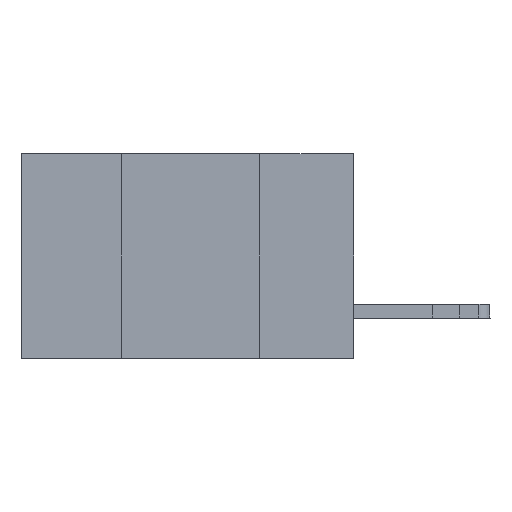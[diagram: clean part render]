
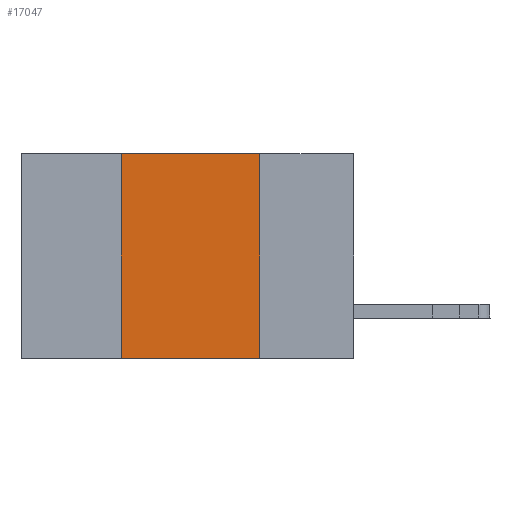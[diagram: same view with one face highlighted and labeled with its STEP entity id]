
A CAD part, left-side view. The second image highlights one B-rep face of the part: STEP entity #17047.
In plain terms, the highlighted planar face has unit normal (-1, 0, 0).
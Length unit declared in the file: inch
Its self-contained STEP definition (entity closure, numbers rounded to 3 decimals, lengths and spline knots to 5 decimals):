
#744 = CARTESIAN_POINT ( 'NONE',  ( 0., 0.42, 0. ) ) ;
#841 = CARTESIAN_POINT ( 'NONE',  ( 0., 0.17, 0. ) ) ;
#2110 = VECTOR ( 'NONE', #11971, 39.37008 ) ;
#2555 = CARTESIAN_POINT ( 'NONE',  ( 0., 0.6, 0. ) ) ;
#3295 = CARTESIAN_POINT ( 'NONE',  ( 0., 0.42, -0.37 ) ) ;
#3347 = FACE_OUTER_BOUND ( 'NONE', #13404, .T. ) ;
#5557 = CARTESIAN_POINT ( 'NONE',  ( 0., 0.42, 0. ) ) ;
#6804 = AXIS2_PLACEMENT_3D ( 'NONE', #13913, #7875, #20965 ) ;
#7807 = EDGE_CURVE ( 'NONE', #8524, #27632, #11743, .T. ) ;
#7875 = DIRECTION ( 'NONE',  ( 1., 0., 0. ) ) ;
#8524 = VERTEX_POINT ( 'NONE', #3295 ) ;
#8963 = DIRECTION ( 'NONE',  ( 0., -1., 0. ) ) ;
#11543 = VERTEX_POINT ( 'NONE', #24212 ) ;
#11629 = DIRECTION ( 'NONE',  ( 0., -1., 0. ) ) ;
#11743 = LINE ( 'NONE', #18337, #21527 ) ;
#11971 = DIRECTION ( 'NONE',  ( 0., 0., -1. ) ) ;
#13344 = EDGE_CURVE ( 'NONE', #11543, #27632, #19985, .T. ) ;
#13404 = EDGE_LOOP ( 'NONE', ( #27558, #22235, #19553, #14468 ) ) ;
#13735 = PLANE ( 'NONE',  #6804 ) ;
#13913 = CARTESIAN_POINT ( 'NONE',  ( 0., 0.6, 0. ) ) ;
#14468 = ORIENTED_EDGE ( 'NONE', *, *, #7807, .T. ) ;
#14737 = EDGE_CURVE ( 'NONE', #17243, #11543, #18023, .T. ) ;
#16225 = DIRECTION ( 'NONE',  ( 0., 0., 1. ) ) ;
#16736 = EDGE_CURVE ( 'NONE', #8524, #17243, #17237, .T. ) ;
#17047 = ADVANCED_FACE ( 'NONE', ( #3347 ), #13735, .F. ) ;
#17237 = LINE ( 'NONE', #744, #18557 ) ;
#17243 = VERTEX_POINT ( 'NONE', #5557 ) ;
#18023 = LINE ( 'NONE', #2555, #20985 ) ;
#18337 = CARTESIAN_POINT ( 'NONE',  ( 0., 0.6, -0.37 ) ) ;
#18557 = VECTOR ( 'NONE', #16225, 39.37008 ) ;
#18874 = CARTESIAN_POINT ( 'NONE',  ( 0., 0.17, -0.37 ) ) ;
#19553 = ORIENTED_EDGE ( 'NONE', *, *, #16736, .F. ) ;
#19985 = LINE ( 'NONE', #841, #2110 ) ;
#20965 = DIRECTION ( 'NONE',  ( 0., 0., -1. ) ) ;
#20985 = VECTOR ( 'NONE', #8963, 39.37008 ) ;
#21527 = VECTOR ( 'NONE', #11629, 39.37008 ) ;
#22235 = ORIENTED_EDGE ( 'NONE', *, *, #14737, .F. ) ;
#24212 = CARTESIAN_POINT ( 'NONE',  ( 0., 0.17, 0. ) ) ;
#27558 = ORIENTED_EDGE ( 'NONE', *, *, #13344, .F. ) ;
#27632 = VERTEX_POINT ( 'NONE', #18874 ) ;
